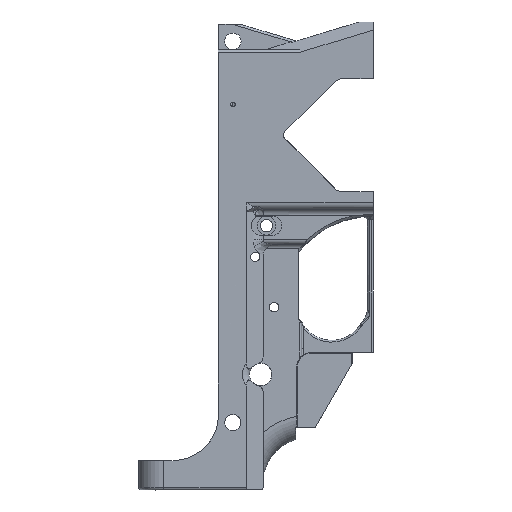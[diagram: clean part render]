
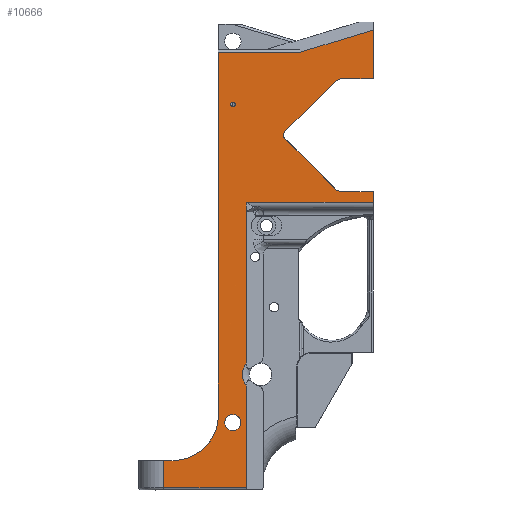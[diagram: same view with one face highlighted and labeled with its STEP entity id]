
A CAD part, left-side view. The second image highlights one B-rep face of the part: STEP entity #10666.
In plain terms, the highlighted planar face has unit normal (-1, 0, 0).
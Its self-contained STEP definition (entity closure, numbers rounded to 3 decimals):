
#93=CARTESIAN_POINT('',(-18.567,27.673,-78.994));
#94=DIRECTION('',(1.,0.,0.));
#95=DIRECTION('',(0.,0.,1.));
#96=AXIS2_PLACEMENT_3D('',#93,#94,#95);
#98=CARTESIAN_POINT('',(-18.567,27.673,-78.994));
#99=DIRECTION('',(1.,0.,0.));
#100=DIRECTION('',(0.,0.,-1.));
#101=AXIS2_PLACEMENT_3D('',#98,#99,#100);
#103=CARTESIAN_POINT('',(-18.567,27.673,56.134));
#104=DIRECTION('',(1.,0.,0.));
#105=DIRECTION('',(0.,1.,0.));
#106=AXIS2_PLACEMENT_3D('',#103,#104,#105);
#108=CARTESIAN_POINT('',(-18.567,27.673,56.134));
#109=DIRECTION('',(1.,0.,0.));
#110=DIRECTION('',(0.,-1.,0.));
#111=AXIS2_PLACEMENT_3D('',#108,#109,#110);
#113=DIRECTION('',(0.,0.,1.));
#114=VECTOR('',#113,64.279);
#115=CARTESIAN_POINT('',(-18.567,21.916,-53.692));
#116=LINE('',#115,#114);
#117=CARTESIAN_POINT('',(-18.567,15.9,-58.598));
#118=DIRECTION('',(1.,0.,0.));
#119=DIRECTION('',(0.,0.775,-0.632));
#120=AXIS2_PLACEMENT_3D('',#117,#118,#119);
#122=DIRECTION('',(0.,0.,-1.));
#123=VECTOR('',#122,43.142);
#124=CARTESIAN_POINT('',(-18.567,21.916,-63.504));
#125=LINE('',#124,#123);
#126=CARTESIAN_POINT('',(-18.567,53.086,-75.819));
#127=DIRECTION('',(1.,0.,0.));
#128=DIRECTION('',(0.,-1.,0.));
#129=AXIS2_PLACEMENT_3D('',#126,#127,#128);
#131=DIRECTION('',(0.,0.,1.));
#132=VECTOR('',#131,154.067);
#133=CARTESIAN_POINT('',(-18.567,33.786,-75.819));
#134=LINE('',#133,#132);
#135=DIRECTION('',(0.,-1.,0.));
#136=VECTOR('',#135,34.547);
#137=CARTESIAN_POINT('',(-18.567,33.786,78.248));
#138=LINE('',#137,#136);
#139=DIRECTION('',(0.,1.,0.));
#140=VECTOR('',#139,14.);
#141=CARTESIAN_POINT('',(-18.567,-32.004,67.005));
#142=LINE('',#141,#140);
#143=DIRECTION('',(0.,-0.707,0.707));
#144=VECTOR('',#143,30.941);
#145=CARTESIAN_POINT('',(-18.567,5.582,44.419));
#146=LINE('',#145,#144);
#147=DIRECTION('',(0.,0.707,0.707));
#148=VECTOR('',#147,30.941);
#149=CARTESIAN_POINT('',(-18.567,-16.297,19.712));
#150=LINE('',#149,#148);
#151=DIRECTION('',(0.,1.,0.));
#152=VECTOR('',#151,14.);
#153=CARTESIAN_POINT('',(-18.567,-32.004,19.005));
#154=LINE('',#153,#152);
#155=DIRECTION('',(0.,0.,-1.));
#156=VECTOR('',#155,4.484);
#157=CARTESIAN_POINT('',(-18.567,-32.004,19.005));
#158=LINE('',#157,#156);
#159=CARTESIAN_POINT('',(-18.565,21.916,14.346));
#160=CARTESIAN_POINT('',(-18.565,21.916,14.366));
#161=CARTESIAN_POINT('',(-18.567,21.916,14.404));
#162=CARTESIAN_POINT('',(-18.566,21.916,14.463));
#163=CARTESIAN_POINT('',(-18.567,21.916,14.501));
#164=CARTESIAN_POINT('',(-18.567,21.916,14.521));
#839=DIRECTION('',(0.,0.957,-0.29));
#840=VECTOR('',#839,32.646);
#841=CARTESIAN_POINT('',(-18.567,-32.004,87.717));
#842=LINE('',#841,#840);
#2586=DIRECTION('',(0.,-1.,0.));
#2587=VECTOR('',#2586,3.965);
#2588=CARTESIAN_POINT('',(-18.567,57.051,-95.119));
#2589=LINE('',#2588,#2587);
#3763=CARTESIAN_POINT('',(-18.567,21.916,
-53.692));
#5980=DIRECTION('',(0.,0.,1.));
#5981=VECTOR('',#5980,20.711);
#5982=CARTESIAN_POINT('',(-18.567,-32.004,67.005));
#5983=LINE('',#5982,#5981);
#6458=CARTESIAN_POINT('',(-18.567,4.168,43.005));
#6459=DIRECTION('',(1.,0.,0.));
#6460=DIRECTION('',(0.,0.707,-0.707));
#6461=AXIS2_PLACEMENT_3D('',#6458,#6459,#6460);
#6467=DIRECTION('',(0.,-0.924,0.383));
#6468=VECTOR('',#6467,1.848);
#6469=CARTESIAN_POINT('',(-18.567,-16.297,
66.298));
#6470=LINE('',#6469,#6468);
#7415=DIRECTION('',(0.,0.924,0.383));
#7416=VECTOR('',#7415,1.848);
#7417=CARTESIAN_POINT('',(-18.567,-18.004,19.005));
#7418=LINE('',#7417,#7416);
#7833=CARTESIAN_POINT('',(-18.565,21.916,14.346));
#7840=DIRECTION('',(0.,-1.,0.));
#7841=VECTOR('',#7840,53.92);
#7842=CARTESIAN_POINT('',(-18.567,21.916,14.521));
#7843=LINE('',#7842,#7841);
#7856=DIRECTION('',(0.,0.,1.));
#7857=VECTOR('',#7856,3.759);
#7858=CARTESIAN_POINT('',(-18.567,21.916,10.587));
#7859=LINE('',#7858,#7857);
#8248=DIRECTION('',(0.,0.,1.));
#8249=VECTOR('',#8248,11.526);
#8250=CARTESIAN_POINT('',(-18.567,57.051,-106.645));
#8251=LINE('',#8250,#8249);
#8279=DIRECTION('',(0.,1.,0.));
#8280=VECTOR('',#8279,35.135);
#8281=CARTESIAN_POINT('',(-18.567,21.916,
-106.645));
#8282=LINE('',#8281,#8280);
#8987=CARTESIAN_POINT('',(-18.567,57.051,-106.645));
#8989=VERTEX_POINT('',#8987);
#9184=CARTESIAN_POINT('',(-18.567,53.086,-95.119));
#9186=VERTEX_POINT('',#9184);
#9328=CARTESIAN_POINT('',(-18.567,57.051,-95.119));
#9330=VERTEX_POINT('',#9328);
#9386=CARTESIAN_POINT('',(-18.567,33.786,-75.819));
#9388=VERTEX_POINT('',#9386);
#9554=VERTEX_POINT('',#7833);
#9556=VERTEX_POINT('',#164);
#9576=CARTESIAN_POINT('',(-18.567,26.683,56.134));
#9578=VERTEX_POINT('',#9576);
#9580=CARTESIAN_POINT('',(-18.567,28.664,56.134));
#9582=VERTEX_POINT('',#9580);
#9615=CARTESIAN_POINT('',(-18.567,27.673,-75.565));
#9617=VERTEX_POINT('',#9615);
#9619=CARTESIAN_POINT('',(-18.567,27.673,-82.423));
#9621=VERTEX_POINT('',#9619);
#9826=CARTESIAN_POINT('',(-18.567,-32.004,14.521));
#9828=VERTEX_POINT('',#9826);
#9884=CARTESIAN_POINT('',(-18.567,21.916,
-63.504));
#9885=CARTESIAN_POINT('',(-18.567,21.916,
-106.645));
#9886=VERTEX_POINT('',#9884);
#9887=VERTEX_POINT('',#9885);
#9893=VERTEX_POINT('',#3763);
#9955=CARTESIAN_POINT('',(-18.567,-32.004,19.005));
#9956=VERTEX_POINT('',#9955);
#9965=CARTESIAN_POINT('',(-18.567,-18.004,19.005));
#9966=VERTEX_POINT('',#9965);
#9967=CARTESIAN_POINT('',(-18.567,-32.004,67.005));
#9968=CARTESIAN_POINT('',(-18.567,-18.004,67.005));
#9969=VERTEX_POINT('',#9967);
#9970=VERTEX_POINT('',#9968);
#9971=CARTESIAN_POINT('',(-18.567,-16.297,
19.712));
#9972=VERTEX_POINT('',#9971);
#9973=CARTESIAN_POINT('',(-18.567,-16.297,
66.298));
#9974=VERTEX_POINT('',#9973);
#9983=CARTESIAN_POINT('',(-18.567,5.582,41.591));
#9984=VERTEX_POINT('',#9983);
#9985=CARTESIAN_POINT('',(-18.567,5.582,44.419));
#9986=VERTEX_POINT('',#9985);
#10118=CARTESIAN_POINT('',(-18.567,-32.004,87.717));
#10119=VERTEX_POINT('',#10118);
#10224=CARTESIAN_POINT('',(-18.567,33.786,78.248));
#10225=CARTESIAN_POINT('',(-18.567,-0.761,78.248));
#10226=VERTEX_POINT('',#10224);
#10227=VERTEX_POINT('',#10225);
#10365=CARTESIAN_POINT('',(-18.567,21.916,10.587));
#10367=VERTEX_POINT('',#10365);
#10604=CARTESIAN_POINT('',(-18.567,21.916,
61.427));
#10605=DIRECTION('',(-1.,0.,0.));
#10606=DIRECTION('',(0.,0.,1.));
#10607=AXIS2_PLACEMENT_3D('',#10604,#10605,#10606);
#10608=PLANE('',#10607);
#10610=ORIENTED_EDGE('',*,*,#10609,.F.);
#10612=ORIENTED_EDGE('',*,*,#10611,.F.);
#10614=ORIENTED_EDGE('',*,*,#10613,.F.);
#10616=ORIENTED_EDGE('',*,*,#10615,.T.);
#10618=ORIENTED_EDGE('',*,*,#10617,.T.);
#10620=ORIENTED_EDGE('',*,*,#10619,.T.);
#10622=ORIENTED_EDGE('',*,*,#10621,.T.);
#10624=ORIENTED_EDGE('',*,*,#10623,.F.);
#10626=ORIENTED_EDGE('',*,*,#10625,.T.);
#10628=ORIENTED_EDGE('',*,*,#10627,.T.);
#10630=ORIENTED_EDGE('',*,*,#10629,.F.);
#10632=ORIENTED_EDGE('',*,*,#10631,.F.);
#10634=ORIENTED_EDGE('',*,*,#10633,.T.);
#10636=ORIENTED_EDGE('',*,*,#10635,.F.);
#10638=ORIENTED_EDGE('',*,*,#10637,.F.);
#10640=ORIENTED_EDGE('',*,*,#10639,.F.);
#10642=ORIENTED_EDGE('',*,*,#10641,.F.);
#10644=ORIENTED_EDGE('',*,*,#10643,.F.);
#10646=ORIENTED_EDGE('',*,*,#10645,.F.);
#10648=ORIENTED_EDGE('',*,*,#10647,.T.);
#10650=ORIENTED_EDGE('',*,*,#10649,.F.);
#10652=ORIENTED_EDGE('',*,*,#10651,.F.);
#10653=EDGE_LOOP('',(#10610,#10612,#10614,#10616,#10618,#10620,#10622,#10624,
#10626,#10628,#10630,#10632,#10634,#10636,#10638,#10640,#10642,#10644,#10646,
#10648,#10650,#10652));
#10654=FACE_OUTER_BOUND('',#10653,.F.);
#10655=ORIENTED_EDGE('',*,*,#10593,.F.);
#10657=ORIENTED_EDGE('',*,*,#10656,.F.);
#10658=EDGE_LOOP('',(#10655,#10657));
#10659=FACE_BOUND('',#10658,.F.);
#10661=ORIENTED_EDGE('',*,*,#10660,.F.);
#10663=ORIENTED_EDGE('',*,*,#10662,.F.);
#10664=EDGE_LOOP('',(#10661,#10663));
#10665=FACE_BOUND('',#10664,.F.);
#10666=ADVANCED_FACE('',(#10654,#10659,#10665),#10608,.T.);
#97=CIRCLE('',#96,3.429);
#102=CIRCLE('',#101,3.429);
#107=CIRCLE('',#106,0.991);
#112=CIRCLE('',#111,0.991);
#121=CIRCLE('',#120,7.763);
#130=CIRCLE('',#129,19.3);
#165=B_SPLINE_CURVE_WITH_KNOTS('',3,(#159,#160,#161,#162,#163,#164),
.UNSPECIFIED.,.F.,.F.,(4,1,1,4),(0.,0.333,0.667,1.),
.UNSPECIFIED.);
#6462=CIRCLE('',#6461,2.);
#10593=EDGE_CURVE('',#9582,#9578,#107,.T.);
#10609=EDGE_CURVE('',#10367,#9554,#7859,.T.);
#10611=EDGE_CURVE('',#9893,#10367,#116,.T.);
#10613=EDGE_CURVE('',#9886,#9893,#121,.T.);
#10615=EDGE_CURVE('',#9886,#9887,#125,.T.);
#10617=EDGE_CURVE('',#9887,#8989,#8282,.T.);
#10619=EDGE_CURVE('',#8989,#9330,#8251,.T.);
#10621=EDGE_CURVE('',#9330,#9186,#2589,.T.);
#10623=EDGE_CURVE('',#9388,#9186,#130,.T.);
#10625=EDGE_CURVE('',#9388,#10226,#134,.T.);
#10627=EDGE_CURVE('',#10226,#10227,#138,.T.);
#10629=EDGE_CURVE('',#10119,#10227,#842,.T.);
#10631=EDGE_CURVE('',#9969,#10119,#5983,.T.);
#10633=EDGE_CURVE('',#9969,#9970,#142,.T.);
#10635=EDGE_CURVE('',#9974,#9970,#6470,.T.);
#10637=EDGE_CURVE('',#9986,#9974,#146,.T.);
#10639=EDGE_CURVE('',#9984,#9986,#6462,.T.);
#10641=EDGE_CURVE('',#9972,#9984,#150,.T.);
#10643=EDGE_CURVE('',#9966,#9972,#7418,.T.);
#10645=EDGE_CURVE('',#9956,#9966,#154,.T.);
#10647=EDGE_CURVE('',#9956,#9828,#158,.T.);
#10649=EDGE_CURVE('',#9556,#9828,#7843,.T.);
#10651=EDGE_CURVE('',#9554,#9556,#165,.T.);
#10656=EDGE_CURVE('',#9578,#9582,#112,.T.);
#10660=EDGE_CURVE('',#9617,#9621,#97,.T.);
#10662=EDGE_CURVE('',#9621,#9617,#102,.T.);
